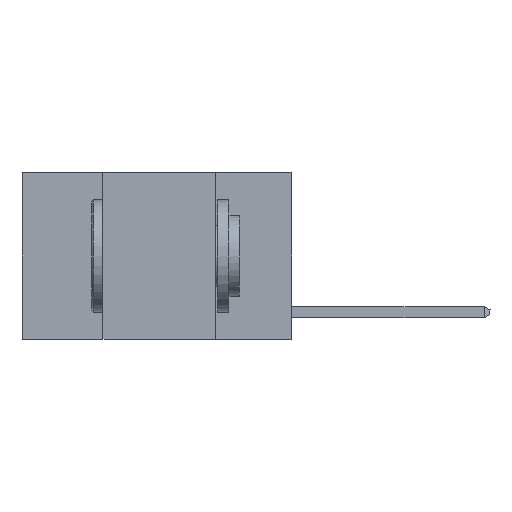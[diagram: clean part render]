
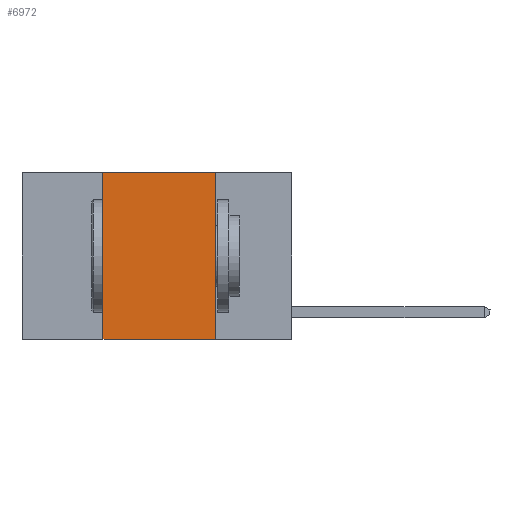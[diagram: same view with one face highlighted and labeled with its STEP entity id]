
A CAD part, left-side view. The second image highlights one B-rep face of the part: STEP entity #6972.
In plain terms, the highlighted planar face has unit normal (-1, 0, 0).
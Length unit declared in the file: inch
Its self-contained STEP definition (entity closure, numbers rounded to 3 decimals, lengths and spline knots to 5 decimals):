
#291 = DIRECTION ( 'NONE',  ( 0., -1., 0. ) ) ;
#1553 = VECTOR ( 'NONE', #26453, 39.37008 ) ;
#2821 = CARTESIAN_POINT ( 'NONE',  ( 0., 0.42, 0. ) ) ;
#3000 = VERTEX_POINT ( 'NONE', #18285 ) ;
#3996 = ORIENTED_EDGE ( 'NONE', *, *, #7559, .F. ) ;
#4492 = EDGE_CURVE ( 'NONE', #3000, #22009, #6470, .T. ) ;
#5645 = AXIS2_PLACEMENT_3D ( 'NONE', #24658, #16323, #14302 ) ;
#6216 = FACE_OUTER_BOUND ( 'NONE', #18559, .T. ) ;
#6470 = LINE ( 'NONE', #2821, #22396 ) ;
#6738 = ORIENTED_EDGE ( 'NONE', *, *, #7143, .T. ) ;
#6972 = ADVANCED_FACE ( 'NONE', ( #6216 ), #22590, .F. ) ;
#7143 = EDGE_CURVE ( 'NONE', #3000, #7914, #22476, .T. ) ;
#7559 = EDGE_CURVE ( 'NONE', #22009, #20978, #19801, .T. ) ;
#7914 = VERTEX_POINT ( 'NONE', #11275 ) ;
#9134 = EDGE_CURVE ( 'NONE', #20978, #7914, #15194, .T. ) ;
#10584 = CARTESIAN_POINT ( 'NONE',  ( 0., 0.6, -0.37 ) ) ;
#11275 = CARTESIAN_POINT ( 'NONE',  ( 0., 0.17, -0.37 ) ) ;
#12379 = ORIENTED_EDGE ( 'NONE', *, *, #4492, .F. ) ;
#12388 = DIRECTION ( 'NONE',  ( 0., -1., 0. ) ) ;
#12821 = ORIENTED_EDGE ( 'NONE', *, *, #9134, .F. ) ;
#14302 = DIRECTION ( 'NONE',  ( 0., 0., -1. ) ) ;
#14956 = CARTESIAN_POINT ( 'NONE',  ( 0., 0.6, 0. ) ) ;
#15194 = LINE ( 'NONE', #18133, #1553 ) ;
#15272 = VECTOR ( 'NONE', #291, 39.37008 ) ;
#15629 = DIRECTION ( 'NONE',  ( 0., 0., 1. ) ) ;
#16323 = DIRECTION ( 'NONE',  ( 1., 0., 0. ) ) ;
#18133 = CARTESIAN_POINT ( 'NONE',  ( 0., 0.17, 0. ) ) ;
#18285 = CARTESIAN_POINT ( 'NONE',  ( 0., 0.42, -0.37 ) ) ;
#18559 = EDGE_LOOP ( 'NONE', ( #12821, #3996, #12379, #6738 ) ) ;
#19801 = LINE ( 'NONE', #14956, #15272 ) ;
#20978 = VERTEX_POINT ( 'NONE', #22853 ) ;
#22009 = VERTEX_POINT ( 'NONE', #24328 ) ;
#22396 = VECTOR ( 'NONE', #15629, 39.37008 ) ;
#22476 = LINE ( 'NONE', #10584, #23424 ) ;
#22590 = PLANE ( 'NONE',  #5645 ) ;
#22853 = CARTESIAN_POINT ( 'NONE',  ( 0., 0.17, 0. ) ) ;
#23424 = VECTOR ( 'NONE', #12388, 39.37008 ) ;
#24328 = CARTESIAN_POINT ( 'NONE',  ( 0., 0.42, 0. ) ) ;
#24658 = CARTESIAN_POINT ( 'NONE',  ( 0., 0.6, 0. ) ) ;
#26453 = DIRECTION ( 'NONE',  ( 0., 0., -1. ) ) ;
